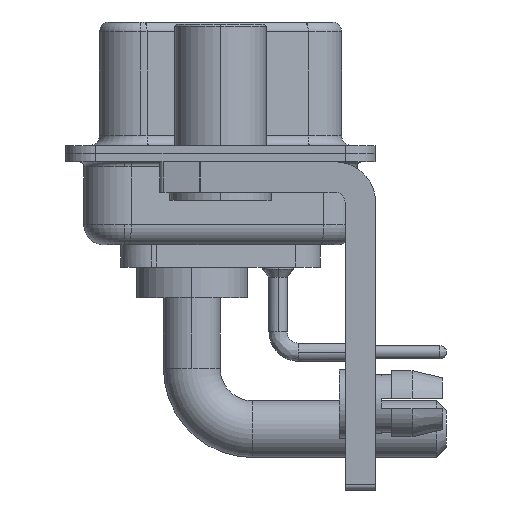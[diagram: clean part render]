
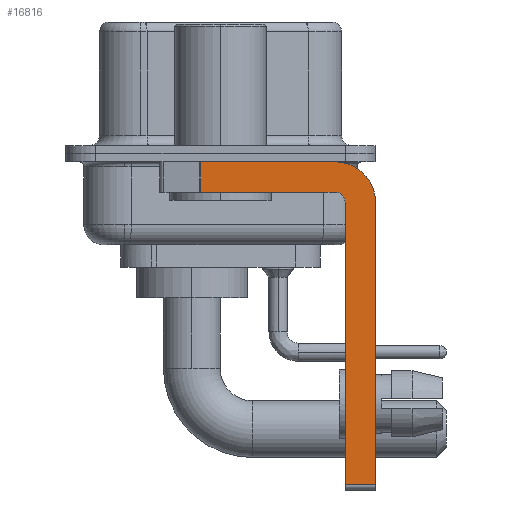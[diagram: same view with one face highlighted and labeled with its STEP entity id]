
A CAD part, left-side view. The second image highlights one B-rep face of the part: STEP entity #16816.
In plain terms, the highlighted planar face has unit normal (-1, 0, 0).
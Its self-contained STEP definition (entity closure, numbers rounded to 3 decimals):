
#425 = ORIENTED_EDGE ( 'NONE', *, *, #664, .F. ) ;
#517 = CARTESIAN_POINT ( 'NONE',  ( -2.9, -6.15, -16.35 ) ) ;
#664 = EDGE_CURVE ( 'NONE', #8447, #15841, #11884, .T. ) ;
#701 = VERTEX_POINT ( 'NONE', #16304 ) ;
#1607 = DIRECTION ( 'NONE',  ( 0., -1., 0. ) ) ;
#1640 = VECTOR ( 'NONE', #16355, 1000. ) ;
#1768 = CARTESIAN_POINT ( 'NONE',  ( -2.9, -6.15, -2.4 ) ) ;
#2828 = CIRCLE ( 'NONE', #17422, 2. ) ;
#2944 = CARTESIAN_POINT ( 'NONE',  ( -2.9, 3., -0.4 ) ) ;
#3167 = ORIENTED_EDGE ( 'NONE', *, *, #21797, .F. ) ;
#3249 = DIRECTION ( 'NONE',  ( 1., 0., 0. ) ) ;
#4512 = CARTESIAN_POINT ( 'NONE',  ( -2.9, -7.65, -16.35 ) ) ;
#5305 = AXIS2_PLACEMENT_3D ( 'NONE', #23382, #12714, #27418 ) ;
#5647 = PLANE ( 'NONE',  #11307 ) ;
#5903 = LINE ( 'NONE', #14088, #20654 ) ;
#5918 = VECTOR ( 'NONE', #16166, 1000. ) ;
#6699 = DIRECTION ( 'NONE',  ( 0., -1., 0. ) ) ;
#7359 = CARTESIAN_POINT ( 'NONE',  ( -2.9, -5.65, -0.4 ) ) ;
#7847 = CARTESIAN_POINT ( 'NONE',  ( -2.9, -5.65, -1.9 ) ) ;
#8170 = CARTESIAN_POINT ( 'NONE',  ( -2.9, -7.65, -2.4 ) ) ;
#8447 = VERTEX_POINT ( 'NONE', #16939 ) ;
#9970 = VERTEX_POINT ( 'NONE', #7359 ) ;
#10117 = EDGE_LOOP ( 'NONE', ( #11459, #13545, #425, #18295, #3167, #13961, #19827, #16897 ) ) ;
#11307 = AXIS2_PLACEMENT_3D ( 'NONE', #18260, #26727, #22425 ) ;
#11315 = LINE ( 'NONE', #15733, #26510 ) ;
#11459 = ORIENTED_EDGE ( 'NONE', *, *, #26563, .F. ) ;
#11884 = LINE ( 'NONE', #7847, #16178 ) ;
#12150 = VERTEX_POINT ( 'NONE', #4512 ) ;
#12329 = EDGE_CURVE ( 'NONE', #9970, #701, #2828, .T. ) ;
#12714 = DIRECTION ( 'NONE',  ( -1., 0., 0. ) ) ;
#12787 = CARTESIAN_POINT ( 'NONE',  ( -2.9, 0.978, -0.4 ) ) ;
#13545 = ORIENTED_EDGE ( 'NONE', *, *, #15593, .T. ) ;
#13557 = FACE_OUTER_BOUND ( 'NONE', #10117, .T. ) ;
#13961 = ORIENTED_EDGE ( 'NONE', *, *, #25787, .T. ) ;
#14088 = CARTESIAN_POINT ( 'NONE',  ( -2.9, -5.65, -16.35 ) ) ;
#14406 = LINE ( 'NONE', #8170, #1640 ) ;
#15593 = EDGE_CURVE ( 'NONE', #19411, #15841, #20335, .T. ) ;
#15733 = CARTESIAN_POINT ( 'NONE',  ( -2.9, -6.15, -16.6 ) ) ;
#15841 = VERTEX_POINT ( 'NONE', #17271 ) ;
#16166 = DIRECTION ( 'NONE',  ( 0., 0., -1. ) ) ;
#16178 = VECTOR ( 'NONE', #27127, 1000. ) ;
#16304 = CARTESIAN_POINT ( 'NONE',  ( -2.9, -7.65, -2.4 ) ) ;
#16355 = DIRECTION ( 'NONE',  ( 0., 0., -1. ) ) ;
#16816 = ADVANCED_FACE ( 'NONE', ( #13557 ), #5647, .F. ) ;
#16897 = ORIENTED_EDGE ( 'NONE', *, *, #12329, .F. ) ;
#16939 = CARTESIAN_POINT ( 'NONE',  ( -2.9, -5.65, -1.9 ) ) ;
#17256 = CIRCLE ( 'NONE', #5305, 0.5 ) ;
#17271 = CARTESIAN_POINT ( 'NONE',  ( -2.9, 0.978, -1.9 ) ) ;
#17422 = AXIS2_PLACEMENT_3D ( 'NONE', #20017, #3249, #21696 ) ;
#18260 = CARTESIAN_POINT ( 'NONE',  ( -2.9, -5.65, -2.4 ) ) ;
#18295 = ORIENTED_EDGE ( 'NONE', *, *, #23041, .F. ) ;
#18422 = EDGE_CURVE ( 'NONE', #701, #12150, #14406, .T. ) ;
#19307 = LINE ( 'NONE', #2944, #22487 ) ;
#19411 = VERTEX_POINT ( 'NONE', #12787 ) ;
#19827 = ORIENTED_EDGE ( 'NONE', *, *, #18422, .F. ) ;
#20017 = CARTESIAN_POINT ( 'NONE',  ( -2.9, -5.65, -2.4 ) ) ;
#20335 = LINE ( 'NONE', #24505, #5918 ) ;
#20654 = VECTOR ( 'NONE', #1607, 1000. ) ;
#21480 = VERTEX_POINT ( 'NONE', #1768 ) ;
#21696 = DIRECTION ( 'NONE',  ( 0., 0., -1. ) ) ;
#21797 = EDGE_CURVE ( 'NONE', #25604, #21480, #11315, .T. ) ;
#22425 = DIRECTION ( 'NONE',  ( 0., 0., -1. ) ) ;
#22487 = VECTOR ( 'NONE', #6699, 1000. ) ;
#23041 = EDGE_CURVE ( 'NONE', #21480, #8447, #17256, .T. ) ;
#23382 = CARTESIAN_POINT ( 'NONE',  ( -2.9, -5.65, -2.4 ) ) ;
#24505 = CARTESIAN_POINT ( 'NONE',  ( -2.9, 0.978, -1.9 ) ) ;
#25604 = VERTEX_POINT ( 'NONE', #517 ) ;
#25787 = EDGE_CURVE ( 'NONE', #25604, #12150, #5903, .T. ) ;
#25880 = DIRECTION ( 'NONE',  ( 0., 0., 1. ) ) ;
#26510 = VECTOR ( 'NONE', #25880, 1000. ) ;
#26563 = EDGE_CURVE ( 'NONE', #19411, #9970, #19307, .T. ) ;
#26727 = DIRECTION ( 'NONE',  ( 1., 0., 0. ) ) ;
#27127 = DIRECTION ( 'NONE',  ( 0., 1., 0. ) ) ;
#27418 = DIRECTION ( 'NONE',  ( 0., 0., 1. ) ) ;
